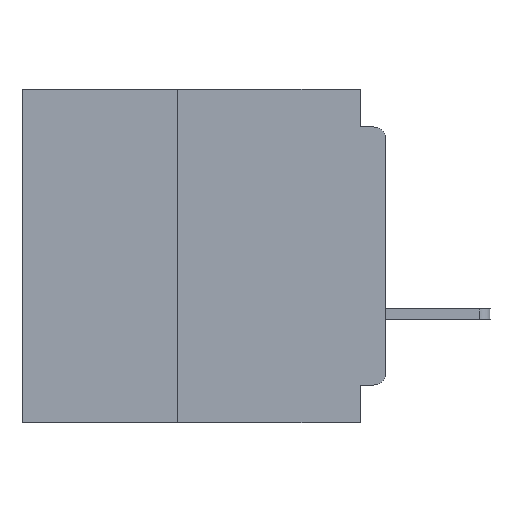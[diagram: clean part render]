
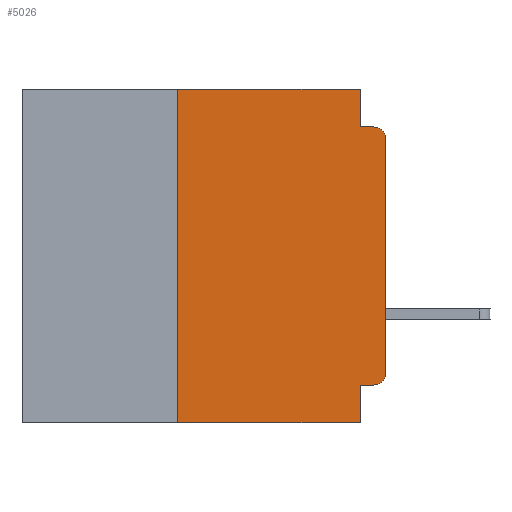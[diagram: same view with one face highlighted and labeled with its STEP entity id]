
A CAD part, left-side view. The second image highlights one B-rep face of the part: STEP entity #5026.
In plain terms, the highlighted planar face has unit normal (-1, 0, 0).
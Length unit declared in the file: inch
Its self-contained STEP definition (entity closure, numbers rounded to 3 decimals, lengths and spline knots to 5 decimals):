
#222 = CARTESIAN_POINT ( 'NONE',  ( 0., 0.031, -0.045 ) ) ;
#2553 = EDGE_CURVE ( 'NONE', #53350, #38627, #30133, .T. ) ;
#2668 = DIRECTION ( 'NONE',  ( 0., 0., -1. ) ) ;
#2762 = AXIS2_PLACEMENT_3D ( 'NONE', #10171, #42593, #14895 ) ;
#2814 = DIRECTION ( 'NONE',  ( 1., 0., 0. ) ) ;
#3236 = CARTESIAN_POINT ( 'NONE',  ( 0., 0.437, 0. ) ) ;
#3250 = DIRECTION ( 'NONE',  ( 0., 0., 1. ) ) ;
#3473 = VECTOR ( 'NONE', #12365, 39.37008 ) ;
#3749 = PLANE ( 'NONE',  #53188 ) ;
#5026 = ADVANCED_FACE ( 'NONE', ( #53718 ), #3749, .F. ) ;
#5809 = EDGE_CURVE ( 'NONE', #10249, #28287, #49433, .T. ) ;
#6086 = ORIENTED_EDGE ( 'NONE', *, *, #20015, .T. ) ;
#6411 = LINE ( 'NONE', #7687, #3473 ) ;
#6942 = ORIENTED_EDGE ( 'NONE', *, *, #5809, .F. ) ;
#7067 = ORIENTED_EDGE ( 'NONE', *, *, #44636, .F. ) ;
#7687 = CARTESIAN_POINT ( 'NONE',  ( 0., 0., 0. ) ) ;
#10171 = CARTESIAN_POINT ( 'NONE',  ( 0., 0.015, -0.06 ) ) ;
#10203 = CARTESIAN_POINT ( 'NONE',  ( 0., 0.031, 0. ) ) ;
#10249 = VERTEX_POINT ( 'NONE', #25261 ) ;
#12365 = DIRECTION ( 'NONE',  ( 0., 0., 1. ) ) ;
#12753 = VECTOR ( 'NONE', #46385, 39.37008 ) ;
#12824 = EDGE_CURVE ( 'NONE', #31632, #53579, #6411, .T. ) ;
#14895 = DIRECTION ( 'NONE',  ( 0., 0., -1. ) ) ;
#15386 = CARTESIAN_POINT ( 'NONE',  ( 0., 0.25, 0. ) ) ;
#15762 = ORIENTED_EDGE ( 'NONE', *, *, #54313, .F. ) ;
#15964 = EDGE_CURVE ( 'NONE', #48657, #39348, #45998, .T. ) ;
#18517 = ORIENTED_EDGE ( 'NONE', *, *, #26846, .F. ) ;
#18608 = ORIENTED_EDGE ( 'NONE', *, *, #40629, .T. ) ;
#18690 = ORIENTED_EDGE ( 'NONE', *, *, #15964, .F. ) ;
#20015 = EDGE_CURVE ( 'NONE', #22747, #38222, #51034, .T. ) ;
#20564 = CARTESIAN_POINT ( 'NONE',  ( 0., 0.015, -0.34 ) ) ;
#20660 = CIRCLE ( 'NONE', #2762, 0.015 ) ;
#21254 = CARTESIAN_POINT ( 'NONE',  ( 0., 0.25, -0.4 ) ) ;
#22747 = VERTEX_POINT ( 'NONE', #21254 ) ;
#22986 = CARTESIAN_POINT ( 'NONE',  ( 0., 0.437, 0. ) ) ;
#23940 = EDGE_CURVE ( 'NONE', #10249, #31632, #38283, .T. ) ;
#25071 = CARTESIAN_POINT ( 'NONE',  ( 0., 0.031, -0.4 ) ) ;
#25261 = CARTESIAN_POINT ( 'NONE',  ( 0., 0.015, -0.355 ) ) ;
#25276 = DIRECTION ( 'NONE',  ( 0., 0., -1. ) ) ;
#26846 = EDGE_CURVE ( 'NONE', #28287, #38222, #52238, .T. ) ;
#27925 = VECTOR ( 'NONE', #38120, 39.37008 ) ;
#28287 = VERTEX_POINT ( 'NONE', #49304 ) ;
#30133 = LINE ( 'NONE', #31867, #54377 ) ;
#31632 = VERTEX_POINT ( 'NONE', #41499 ) ;
#31801 = DIRECTION ( 'NONE',  ( 0., -1., 0. ) ) ;
#31867 = CARTESIAN_POINT ( 'NONE',  ( 0., 0., -0.045 ) ) ;
#31915 = VECTOR ( 'NONE', #3250, 39.37008 ) ;
#33333 = LINE ( 'NONE', #54043, #31915 ) ;
#33897 = VECTOR ( 'NONE', #46101, 39.37008 ) ;
#35236 = AXIS2_PLACEMENT_3D ( 'NONE', #20564, #52737, #25276 ) ;
#37348 = VECTOR ( 'NONE', #41795, 39.37008 ) ;
#37372 = CARTESIAN_POINT ( 'NONE',  ( 0., 0.015, -0.045 ) ) ;
#38120 = DIRECTION ( 'NONE',  ( 0., 0., -1. ) ) ;
#38222 = VERTEX_POINT ( 'NONE', #25071 ) ;
#38283 = CIRCLE ( 'NONE', #35236, 0.015 ) ;
#38627 = VERTEX_POINT ( 'NONE', #37372 ) ;
#39348 = VERTEX_POINT ( 'NONE', #10203 ) ;
#40318 = ORIENTED_EDGE ( 'NONE', *, *, #2553, .F. ) ;
#40558 = ORIENTED_EDGE ( 'NONE', *, *, #12824, .T. ) ;
#40629 = EDGE_CURVE ( 'NONE', #53579, #38627, #20660, .T. ) ;
#41499 = CARTESIAN_POINT ( 'NONE',  ( 0., 0., -0.34 ) ) ;
#41795 = DIRECTION ( 'NONE',  ( 0., 1., 0. ) ) ;
#41932 = CARTESIAN_POINT ( 'NONE',  ( 0., 0., -0.355 ) ) ;
#42593 = DIRECTION ( 'NONE',  ( -1., 0., 0. ) ) ;
#44636 = EDGE_CURVE ( 'NONE', #39348, #53350, #52206, .T. ) ;
#44713 = CARTESIAN_POINT ( 'NONE',  ( 0., 0., -0.06 ) ) ;
#45998 = LINE ( 'NONE', #22986, #33897 ) ;
#46101 = DIRECTION ( 'NONE',  ( 0., -1., 0. ) ) ;
#46385 = DIRECTION ( 'NONE',  ( 0., -1., 0. ) ) ;
#47576 = EDGE_LOOP ( 'NONE', ( #40558, #18608, #40318, #7067, #18690, #15762, #6086, #18517, #6942, #54823 ) ) ;
#48657 = VERTEX_POINT ( 'NONE', #15386 ) ;
#49304 = CARTESIAN_POINT ( 'NONE',  ( 0., 0.031, -0.355 ) ) ;
#49338 = VECTOR ( 'NONE', #57813, 39.37008 ) ;
#49433 = LINE ( 'NONE', #41932, #37348 ) ;
#51034 = LINE ( 'NONE', #51170, #12753 ) ;
#51170 = CARTESIAN_POINT ( 'NONE',  ( 0., 0.437, -0.4 ) ) ;
#51839 = CARTESIAN_POINT ( 'NONE',  ( 0., 0.031, -0.4 ) ) ;
#52206 = LINE ( 'NONE', #53283, #49338 ) ;
#52238 = LINE ( 'NONE', #51839, #27925 ) ;
#52737 = DIRECTION ( 'NONE',  ( -1., 0., 0. ) ) ;
#53188 = AXIS2_PLACEMENT_3D ( 'NONE', #3236, #2814, #2668 ) ;
#53283 = CARTESIAN_POINT ( 'NONE',  ( 0., 0.031, 0. ) ) ;
#53350 = VERTEX_POINT ( 'NONE', #222 ) ;
#53579 = VERTEX_POINT ( 'NONE', #44713 ) ;
#53718 = FACE_OUTER_BOUND ( 'NONE', #47576, .T. ) ;
#54043 = CARTESIAN_POINT ( 'NONE',  ( 0., 0.25, -0.4 ) ) ;
#54313 = EDGE_CURVE ( 'NONE', #22747, #48657, #33333, .T. ) ;
#54377 = VECTOR ( 'NONE', #31801, 39.37008 ) ;
#54823 = ORIENTED_EDGE ( 'NONE', *, *, #23940, .T. ) ;
#57813 = DIRECTION ( 'NONE',  ( 0., 0., -1. ) ) ;
